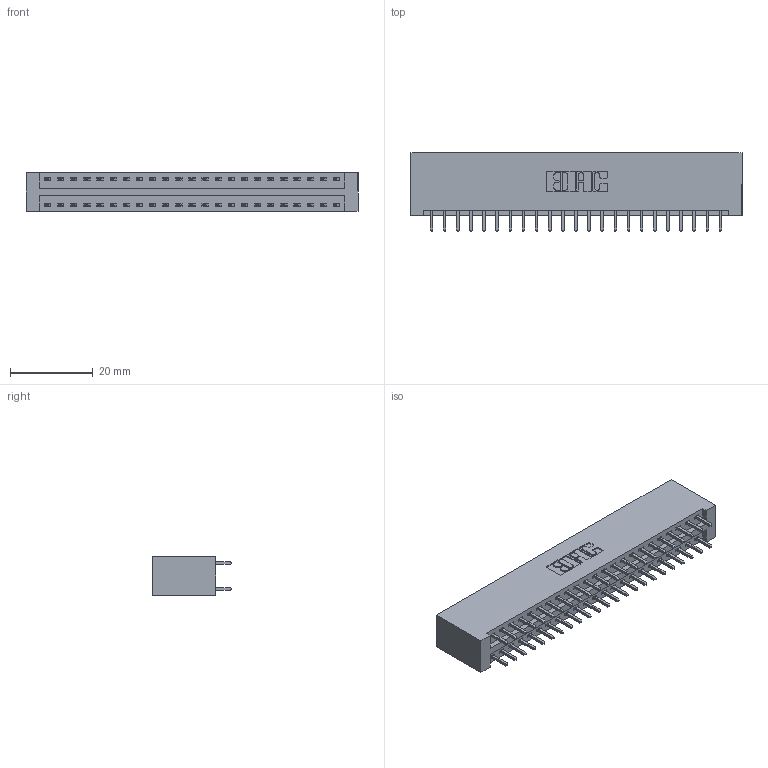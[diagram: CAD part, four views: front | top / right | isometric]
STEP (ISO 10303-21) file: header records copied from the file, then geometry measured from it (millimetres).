
FILE_DESCRIPTION (( 'STEP AP203' ), '1' );
FILE_NAME ('346-046-521-201.STEP', '2018-08-25T04:53:02', ( '' ), ( '' ), 'SwSTEP 2.0', 'SolidWorks 2016', '' );
FILE_SCHEMA (( 'CONFIG_CONTROL_DESIGN' ));
Length unit declared in the file: inch
Products named in the file (3): 346-046-521-201; 346 Part_No Mounting Lugs; 345-292-001_345-293-121
Assembly tree (47 placements, depth 2):
  346-046-521-201
    346 Part_No Mounting Lugs
    345-292-001_345-293-121  x46
Bounding box: 80.26 x 19.05 x 9.4 mm (x, y, z)
Volume: 8233.7 mm3; surface area: 11055.9 mm2
Topology: 47 solids, 47 shells, 2506 faces, 7435 edges, 4894 vertices
Faces by surface type: plane 1682, cylinder 824
Entity records: 17309 total; most frequent: CARTESIAN_POINT 2876, ORIENTED_EDGE 2810, DIRECTION 2581, EDGE_CURVE 1405, LINE 1189, VECTOR 1189, VERTEX_POINT 934, AXIS2_PLACEMENT_3D 696
